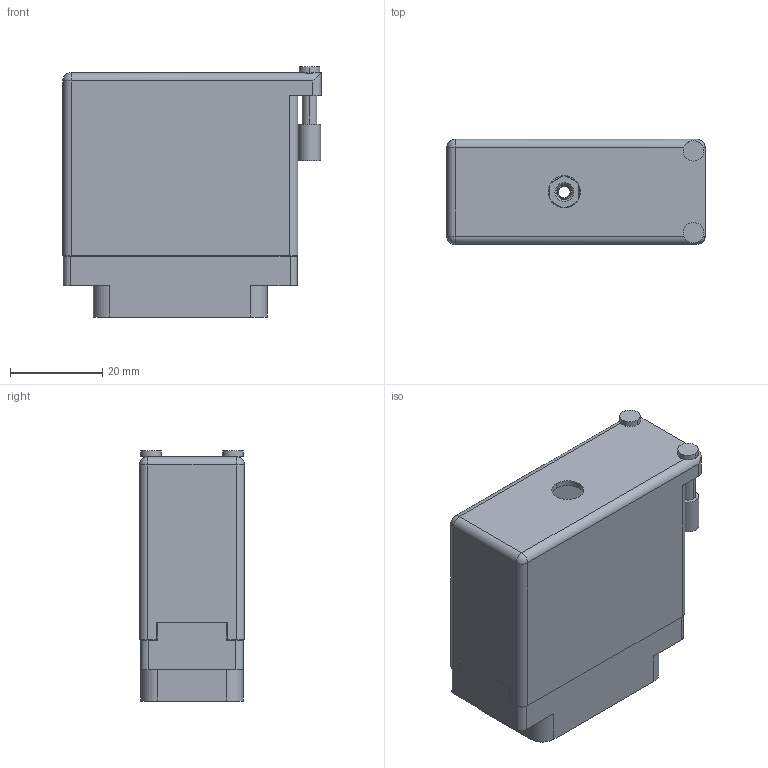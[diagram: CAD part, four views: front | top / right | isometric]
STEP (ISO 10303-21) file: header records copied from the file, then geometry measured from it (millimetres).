
FILE_DESCRIPTION (( 'STEP AP203' ), '1' );
FILE_NAME ('516-038-000-556.STEP', '2020-03-09T19:03:49', ( '' ), ( '' ), 'SwSTEP 2.0', 'SolidWorks 2016', '' );
FILE_SCHEMA (( 'CONFIG_CONTROL_DESIGN' ));
Length unit declared in the file: inch
Products named in the file (4): 516-038-000-556; 516 Plug Insulator_038; 516-252-035-100_516-252-035-100; 516-230-001_Metal - 038 Side Entry
Assembly tree (3 placements, depth 2):
  516-038-000-556
    516 Plug Insulator_038
    516-230-001_Metal - 038 Side Entry
    516-252-035-100_516-252-035-100
Bounding box: 56.08 x 22.83 x 54.31 mm (x, y, z)
Volume: 17573.3 mm3; surface area: 25349.9 mm2
Topology: 3 solids, 3 shells, 1001 faces, 2905 edges, 1928 vertices
Faces by surface type: plane 685, cylinder 296, cone 12, bspline 6, sphere 2
Entity records: 35909 total; most frequent: CARTESIAN_POINT 8325, ORIENTED_EDGE 5806, DIRECTION 5579, EDGE_CURVE 2903, LINE 2119, VECTOR 2119, VERTEX_POINT 1928, AXIS2_PLACEMENT_3D 1730
